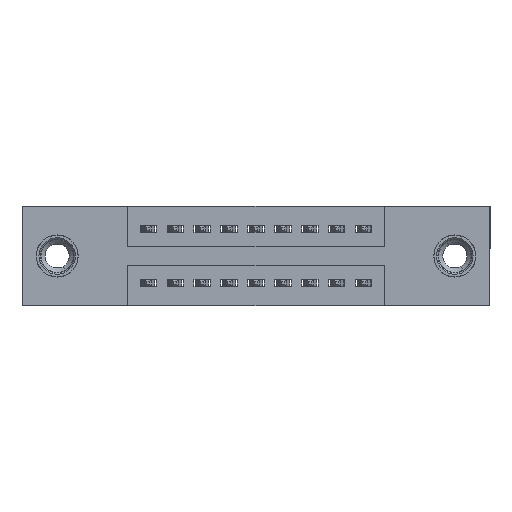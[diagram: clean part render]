
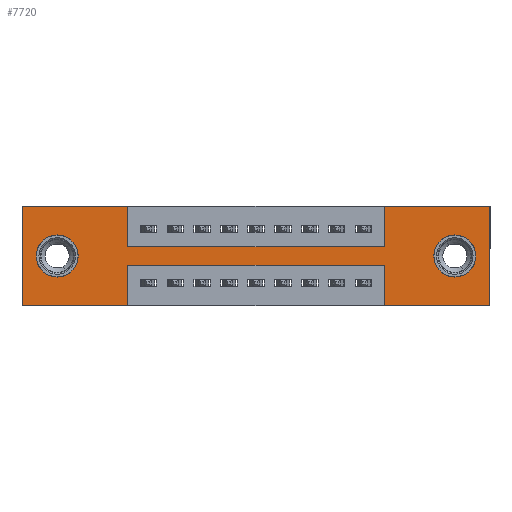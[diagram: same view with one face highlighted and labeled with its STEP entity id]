
A CAD part, front view. The second image highlights one B-rep face of the part: STEP entity #7720.
In plain terms, the highlighted planar face has unit normal (0, -1, 0).
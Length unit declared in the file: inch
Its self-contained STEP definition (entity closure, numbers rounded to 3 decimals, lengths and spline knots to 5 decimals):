
#185 = DIRECTION ( 'NONE',  ( 1., 0., 0. ) ) ;
#212 = VERTEX_POINT ( 'NONE', #5722 ) ;
#231 = VERTEX_POINT ( 'NONE', #3774 ) ;
#235 = ORIENTED_EDGE ( 'NONE', *, *, #10994, .F. ) ;
#286 = CARTESIAN_POINT ( 'NONE',  ( 1.605, 0., -0.185 ) ) ;
#456 = CARTESIAN_POINT ( 'NONE',  ( 1.605, 0., -0.107 ) ) ;
#485 = EDGE_CURVE ( 'NONE', #4756, #11953, #1180, .T. ) ;
#578 = VECTOR ( 'NONE', #10888, 39.37008 ) ;
#1180 = LINE ( 'NONE', #9576, #10466 ) ;
#1201 = VERTEX_POINT ( 'NONE', #456 ) ;
#1234 = VECTOR ( 'NONE', #5093, 39.37008 ) ;
#1236 = ORIENTED_EDGE ( 'NONE', *, *, #485, .F. ) ;
#1248 = CARTESIAN_POINT ( 'NONE',  ( 0.3925, 0., -0.15 ) ) ;
#1396 = VERTEX_POINT ( 'NONE', #4535 ) ;
#1676 = DIRECTION ( 'NONE',  ( 0., 0., -1. ) ) ;
#1702 = CIRCLE ( 'NONE', #4179, 0.078 ) ;
#1732 = LINE ( 'NONE', #9592, #3732 ) ;
#1764 = ORIENTED_EDGE ( 'NONE', *, *, #4727, .F. ) ;
#1872 = AXIS2_PLACEMENT_3D ( 'NONE', #4245, #6461, #6380 ) ;
#1885 = VERTEX_POINT ( 'NONE', #2681 ) ;
#1956 = CARTESIAN_POINT ( 'NONE',  ( 0., 0., 0. ) ) ;
#2042 = ORIENTED_EDGE ( 'NONE', *, *, #5354, .F. ) ;
#2061 = ORIENTED_EDGE ( 'NONE', *, *, #7442, .F. ) ;
#2098 = ORIENTED_EDGE ( 'NONE', *, *, #10136, .F. ) ;
#2119 = ORIENTED_EDGE ( 'NONE', *, *, #10103, .F. ) ;
#2123 = VECTOR ( 'NONE', #9428, 39.37008 ) ;
#2199 = CARTESIAN_POINT ( 'NONE',  ( 0., 0., -0.37 ) ) ;
#2397 = VECTOR ( 'NONE', #6627, 39.37008 ) ;
#2681 = CARTESIAN_POINT ( 'NONE',  ( 0., 0., 0. ) ) ;
#2870 = LINE ( 'NONE', #6965, #8029 ) ;
#2898 = ORIENTED_EDGE ( 'NONE', *, *, #12007, .T. ) ;
#3117 = FACE_BOUND ( 'NONE', #5146, .T. ) ;
#3122 = CARTESIAN_POINT ( 'NONE',  ( 0.3925, 0., -0.22 ) ) ;
#3191 = CARTESIAN_POINT ( 'NONE',  ( 1.735, 0., 0. ) ) ;
#3275 = VERTEX_POINT ( 'NONE', #8909 ) ;
#3391 = LINE ( 'NONE', #12271, #10537 ) ;
#3447 = DIRECTION ( 'NONE',  ( 0., 1., 0. ) ) ;
#3465 = DIRECTION ( 'NONE',  ( 0., 0., -1. ) ) ;
#3596 = CARTESIAN_POINT ( 'NONE',  ( 1.735, 0., -0.37 ) ) ;
#3704 = EDGE_CURVE ( 'NONE', #1201, #3275, #13050, .T. ) ;
#3732 = VECTOR ( 'NONE', #8755, 39.37008 ) ;
#3774 = CARTESIAN_POINT ( 'NONE',  ( 0., 0., -0.37 ) ) ;
#4179 = AXIS2_PLACEMENT_3D ( 'NONE', #286, #13223, #5668 ) ;
#4245 = CARTESIAN_POINT ( 'NONE',  ( 0., 0., -0.37 ) ) ;
#4535 = CARTESIAN_POINT ( 'NONE',  ( 0.13, 0., -0.263 ) ) ;
#4602 = VERTEX_POINT ( 'NONE', #10328 ) ;
#4614 = LINE ( 'NONE', #7184, #7954 ) ;
#4675 = ORIENTED_EDGE ( 'NONE', *, *, #5728, .T. ) ;
#4683 = LINE ( 'NONE', #2199, #13488 ) ;
#4695 = CARTESIAN_POINT ( 'NONE',  ( 0.13, 0., -0.185 ) ) ;
#4727 = EDGE_CURVE ( 'NONE', #4602, #231, #1732, .T. ) ;
#4756 = VERTEX_POINT ( 'NONE', #1248 ) ;
#4921 = EDGE_CURVE ( 'NONE', #10372, #6714, #3391, .T. ) ;
#4975 = VERTEX_POINT ( 'NONE', #13669 ) ;
#5093 = DIRECTION ( 'NONE',  ( 0., 0., -1. ) ) ;
#5140 = CARTESIAN_POINT ( 'NONE',  ( 0.3925, 0., -0.37 ) ) ;
#5146 = EDGE_LOOP ( 'NONE', ( #10397, #2898 ) ) ;
#5354 = EDGE_CURVE ( 'NONE', #11953, #4975, #9354, .T. ) ;
#5527 = EDGE_CURVE ( 'NONE', #212, #1396, #9344, .T. ) ;
#5579 = EDGE_CURVE ( 'NONE', #1885, #11379, #2870, .T. ) ;
#5668 = DIRECTION ( 'NONE',  ( 0., 0., -1. ) ) ;
#5722 = CARTESIAN_POINT ( 'NONE',  ( 0.13, 0., -0.107 ) ) ;
#5728 = EDGE_CURVE ( 'NONE', #3275, #1201, #1702, .T. ) ;
#5780 = CARTESIAN_POINT ( 'NONE',  ( 1.3425, 0., -0.37 ) ) ;
#5849 = CARTESIAN_POINT ( 'NONE',  ( 1.3425, 0., -0.22 ) ) ;
#5892 = CARTESIAN_POINT ( 'NONE',  ( 1.605, 0., -0.185 ) ) ;
#5945 = DIRECTION ( 'NONE',  ( 0., 0., 1. ) ) ;
#6267 = FACE_OUTER_BOUND ( 'NONE', #9695, .T. ) ;
#6369 = DIRECTION ( 'NONE',  ( 0., 0., 1. ) ) ;
#6380 = DIRECTION ( 'NONE',  ( 0., 0., -1. ) ) ;
#6461 = DIRECTION ( 'NONE',  ( 0., -1., 0. ) ) ;
#6627 = DIRECTION ( 'NONE',  ( 0., 0., 1. ) ) ;
#6643 = DIRECTION ( 'NONE',  ( 1., 0., 0. ) ) ;
#6714 = VERTEX_POINT ( 'NONE', #3122 ) ;
#6870 = LINE ( 'NONE', #9875, #8024 ) ;
#6965 = CARTESIAN_POINT ( 'NONE',  ( 0., 0., 0. ) ) ;
#7098 = VERTEX_POINT ( 'NONE', #9347 ) ;
#7184 = CARTESIAN_POINT ( 'NONE',  ( 1.3425, 0., -0.37 ) ) ;
#7442 = EDGE_CURVE ( 'NONE', #9154, #10372, #4614, .T. ) ;
#7720 = ADVANCED_FACE ( 'NONE', ( #9267, #3117, #6267 ), #10604, .T. ) ;
#7954 = VECTOR ( 'NONE', #5945, 39.37008 ) ;
#8024 = VECTOR ( 'NONE', #3465, 39.37008 ) ;
#8029 = VECTOR ( 'NONE', #6643, 39.37008 ) ;
#8034 = LINE ( 'NONE', #3191, #578 ) ;
#8035 = ORIENTED_EDGE ( 'NONE', *, *, #4921, .F. ) ;
#8305 = ORIENTED_EDGE ( 'NONE', *, *, #10250, .F. ) ;
#8743 = ORIENTED_EDGE ( 'NONE', *, *, #10750, .F. ) ;
#8755 = DIRECTION ( 'NONE',  ( -1., 0., 0. ) ) ;
#8909 = CARTESIAN_POINT ( 'NONE',  ( 1.605, 0., -0.263 ) ) ;
#8970 = DIRECTION ( 'NONE',  ( 0., 0., 1. ) ) ;
#9017 = DIRECTION ( 'NONE',  ( 0., 1., 0. ) ) ;
#9154 = VERTEX_POINT ( 'NONE', #5780 ) ;
#9194 = VECTOR ( 'NONE', #6369, 39.37008 ) ;
#9262 = ORIENTED_EDGE ( 'NONE', *, *, #3704, .T. ) ;
#9267 = FACE_BOUND ( 'NONE', #10418, .T. ) ;
#9325 = AXIS2_PLACEMENT_3D ( 'NONE', #5892, #10188, #1676 ) ;
#9344 = CIRCLE ( 'NONE', #11018, 0.078 ) ;
#9347 = CARTESIAN_POINT ( 'NONE',  ( 1.735, 0., 0. ) ) ;
#9354 = LINE ( 'NONE', #9920, #9194 ) ;
#9361 = LINE ( 'NONE', #12980, #2397 ) ;
#9428 = DIRECTION ( 'NONE',  ( 1., 0., 0. ) ) ;
#9576 = CARTESIAN_POINT ( 'NONE',  ( 0.3925, 0., -0.15 ) ) ;
#9592 = CARTESIAN_POINT ( 'NONE',  ( 0., 0., -0.37 ) ) ;
#9695 = EDGE_LOOP ( 'NONE', ( #2119, #8035, #2061, #8743, #2098, #12848, #2042, #1236, #235, #12608, #8305, #1764 ) ) ;
#9803 = DIRECTION ( 'NONE',  ( 0., 0., 1. ) ) ;
#9875 = CARTESIAN_POINT ( 'NONE',  ( 0.3925, 0., 0. ) ) ;
#9920 = CARTESIAN_POINT ( 'NONE',  ( 1.3425, 0., 0. ) ) ;
#10103 = EDGE_CURVE ( 'NONE', #6714, #4602, #12172, .T. ) ;
#10136 = EDGE_CURVE ( 'NONE', #7098, #12000, #8034, .T. ) ;
#10188 = DIRECTION ( 'NONE',  ( 0., 1., 0. ) ) ;
#10250 = EDGE_CURVE ( 'NONE', #231, #1885, #9361, .T. ) ;
#10328 = CARTESIAN_POINT ( 'NONE',  ( 0.3925, 0., -0.37 ) ) ;
#10372 = VERTEX_POINT ( 'NONE', #5849 ) ;
#10397 = ORIENTED_EDGE ( 'NONE', *, *, #5527, .T. ) ;
#10418 = EDGE_LOOP ( 'NONE', ( #9262, #4675 ) ) ;
#10466 = VECTOR ( 'NONE', #185, 39.37008 ) ;
#10537 = VECTOR ( 'NONE', #13400, 39.37008 ) ;
#10604 = PLANE ( 'NONE',  #1872 ) ;
#10750 = EDGE_CURVE ( 'NONE', #12000, #9154, #4683, .T. ) ;
#10888 = DIRECTION ( 'NONE',  ( 0., 0., -1. ) ) ;
#10994 = EDGE_CURVE ( 'NONE', #11379, #4756, #6870, .T. ) ;
#11018 = AXIS2_PLACEMENT_3D ( 'NONE', #12017, #3447, #9803 ) ;
#11379 = VERTEX_POINT ( 'NONE', #12915 ) ;
#11696 = DIRECTION ( 'NONE',  ( -1., 0., 0. ) ) ;
#11837 = CARTESIAN_POINT ( 'NONE',  ( 1.3425, 0., -0.15 ) ) ;
#11953 = VERTEX_POINT ( 'NONE', #11837 ) ;
#12000 = VERTEX_POINT ( 'NONE', #3596 ) ;
#12007 = EDGE_CURVE ( 'NONE', #1396, #212, #12635, .T. ) ;
#12017 = CARTESIAN_POINT ( 'NONE',  ( 0.13, 0., -0.185 ) ) ;
#12107 = AXIS2_PLACEMENT_3D ( 'NONE', #4695, #9017, #8970 ) ;
#12172 = LINE ( 'NONE', #5140, #1234 ) ;
#12229 = LINE ( 'NONE', #1956, #2123 ) ;
#12271 = CARTESIAN_POINT ( 'NONE',  ( 0.3925, 0., -0.22 ) ) ;
#12608 = ORIENTED_EDGE ( 'NONE', *, *, #5579, .F. ) ;
#12635 = CIRCLE ( 'NONE', #12107, 0.078 ) ;
#12668 = EDGE_CURVE ( 'NONE', #4975, #7098, #12229, .T. ) ;
#12848 = ORIENTED_EDGE ( 'NONE', *, *, #12668, .F. ) ;
#12915 = CARTESIAN_POINT ( 'NONE',  ( 0.3925, 0., 0. ) ) ;
#12980 = CARTESIAN_POINT ( 'NONE',  ( 0., 0., 0. ) ) ;
#13050 = CIRCLE ( 'NONE', #9325, 0.078 ) ;
#13223 = DIRECTION ( 'NONE',  ( 0., 1., 0. ) ) ;
#13400 = DIRECTION ( 'NONE',  ( -1., 0., 0. ) ) ;
#13488 = VECTOR ( 'NONE', #11696, 39.37008 ) ;
#13669 = CARTESIAN_POINT ( 'NONE',  ( 1.3425, 0., 0. ) ) ;
